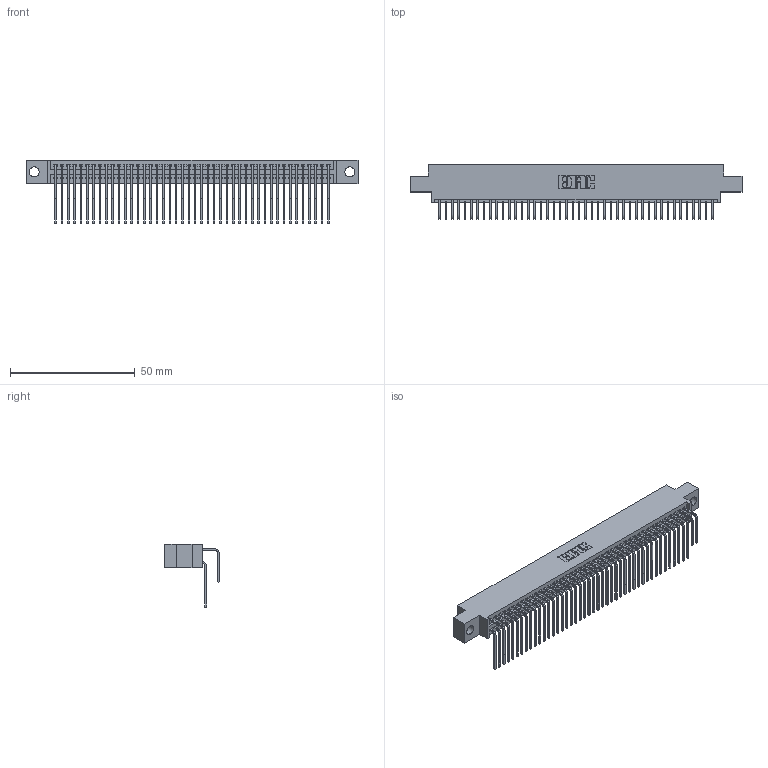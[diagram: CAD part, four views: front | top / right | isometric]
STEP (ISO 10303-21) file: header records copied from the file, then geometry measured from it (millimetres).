
FILE_DESCRIPTION (( 'STEP AP203' ), '1' );
FILE_NAME ('395-088-558-804.STEP', '2021-06-17T09:46:23', ( '' ), ( '' ), 'SwSTEP 2.0', 'SolidWorks 2020', '' );
FILE_SCHEMA (( 'CONFIG_CONTROL_DESIGN' ));
Length unit declared in the file: inch
Products named in the file (4): 345-292-001_558 559 Tail - 1; 395-088-558-804; 345-292-001_558 Tail - 2; 345 Part_0.170 Offset - 0.156 Dia-TI
Assembly tree (89 placements, depth 2):
  395-088-558-804
    345 Part_0.170 Offset - 0.156 Dia-TI
    345-292-001_558 559 Tail - 1  x44
    345-292-001_558 Tail - 2  x44
Bounding box: 132.97 x 21.83 x 25.53 mm (x, y, z)
Volume: 13223.6 mm3; surface area: 21967.7 mm2
Topology: 89 solids, 89 shells, 4720 faces, 14029 edges, 9234 vertices
Faces by surface type: plane 3178, cylinder 1542
Entity records: 36457 total; most frequent: CARTESIAN_POINT 6161, ORIENTED_EDGE 6042, DIRECTION 5401, EDGE_CURVE 3021, LINE 2673, VECTOR 2673, VERTEX_POINT 2010, AXIS2_PLACEMENT_3D 1364
